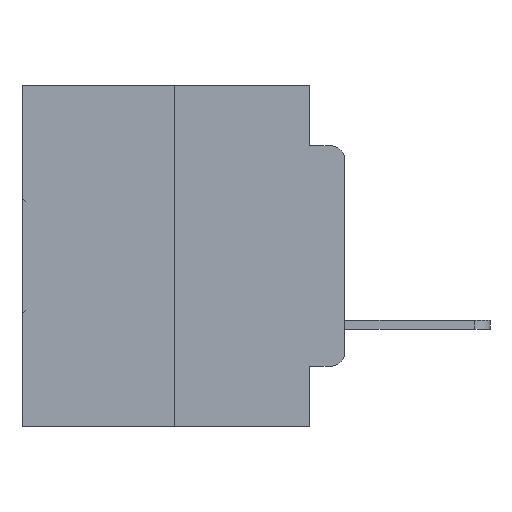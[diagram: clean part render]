
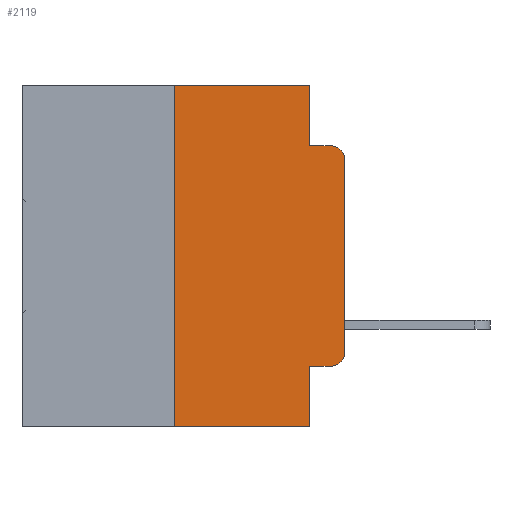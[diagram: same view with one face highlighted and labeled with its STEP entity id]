
A CAD part, left-side view. The second image highlights one B-rep face of the part: STEP entity #2119.
In plain terms, the highlighted planar face has unit normal (-1, 0, 0).
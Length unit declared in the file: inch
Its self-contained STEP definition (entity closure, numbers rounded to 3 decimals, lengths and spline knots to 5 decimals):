
#220 = EDGE_CURVE ( 'NONE', #20294, #27347, #25551, .T. ) ;
#278 = VECTOR ( 'NONE', #11086, 39.37008 ) ;
#612 = EDGE_CURVE ( 'NONE', #7777, #18776, #693, .T. ) ;
#693 = LINE ( 'NONE', #14275, #8654 ) ;
#1566 = LINE ( 'NONE', #29173, #8666 ) ;
#1867 = CARTESIAN_POINT ( 'NONE',  ( 0., 0.473, -0.5 ) ) ;
#1983 = LINE ( 'NONE', #27248, #14309 ) ;
#2119 = ADVANCED_FACE ( 'NONE', ( #10458 ), #27737, .F. ) ;
#2633 = ORIENTED_EDGE ( 'NONE', *, *, #30457, .T. ) ;
#2871 = LINE ( 'NONE', #1867, #22250 ) ;
#3010 = ORIENTED_EDGE ( 'NONE', *, *, #19916, .T. ) ;
#3434 = ORIENTED_EDGE ( 'NONE', *, *, #19320, .T. ) ;
#3666 = CIRCLE ( 'NONE', #27419, 0.02 ) ;
#3745 = CARTESIAN_POINT ( 'NONE',  ( 0., 0.25, 0. ) ) ;
#4259 = EDGE_CURVE ( 'NONE', #26759, #20294, #1566, .T. ) ;
#4433 = CARTESIAN_POINT ( 'NONE',  ( 0., 0.02, -0.1085 ) ) ;
#6158 = VERTEX_POINT ( 'NONE', #17985 ) ;
#6359 = DIRECTION ( 'NONE',  ( 0., -1., 0. ) ) ;
#6365 = ORIENTED_EDGE ( 'NONE', *, *, #220, .F. ) ;
#6709 = VERTEX_POINT ( 'NONE', #20339 ) ;
#7135 = DIRECTION ( 'NONE',  ( 0., 0., -1. ) ) ;
#7457 = CARTESIAN_POINT ( 'NONE',  ( 0., 0.051, -0.0885 ) ) ;
#7753 = DIRECTION ( 'NONE',  ( 0., 0., -1. ) ) ;
#7777 = VERTEX_POINT ( 'NONE', #27759 ) ;
#7784 = VERTEX_POINT ( 'NONE', #30035 ) ;
#8039 = ORIENTED_EDGE ( 'NONE', *, *, #15275, .T. ) ;
#8344 = DIRECTION ( 'NONE',  ( 1., 0., 0. ) ) ;
#8654 = VECTOR ( 'NONE', #7753, 39.37008 ) ;
#8666 = VECTOR ( 'NONE', #31426, 39.37008 ) ;
#10458 = FACE_OUTER_BOUND ( 'NONE', #30214, .T. ) ;
#11080 = CARTESIAN_POINT ( 'NONE',  ( 0., 0.473, 0. ) ) ;
#11086 = DIRECTION ( 'NONE',  ( 0., -1., 0. ) ) ;
#11135 = DIRECTION ( 'NONE',  ( -1., 0., 0. ) ) ;
#12658 = AXIS2_PLACEMENT_3D ( 'NONE', #23118, #8344, #25507 ) ;
#13419 = DIRECTION ( 'NONE',  ( 0., -1., 0. ) ) ;
#13485 = AXIS2_PLACEMENT_3D ( 'NONE', #4433, #22061, #7135 ) ;
#14275 = CARTESIAN_POINT ( 'NONE',  ( 0., 0.051, 0. ) ) ;
#14309 = VECTOR ( 'NONE', #29517, 39.37008 ) ;
#14893 = ORIENTED_EDGE ( 'NONE', *, *, #612, .F. ) ;
#15275 = EDGE_CURVE ( 'NONE', #26759, #18776, #2871, .T. ) ;
#15345 = VERTEX_POINT ( 'NONE', #7457 ) ;
#17192 = CARTESIAN_POINT ( 'NONE',  ( 0., 0.02, -0.4115 ) ) ;
#17556 = ORIENTED_EDGE ( 'NONE', *, *, #23241, .T. ) ;
#17985 = CARTESIAN_POINT ( 'NONE',  ( 0., 0.02, -0.0885 ) ) ;
#18318 = ORIENTED_EDGE ( 'NONE', *, *, #21848, .F. ) ;
#18385 = VECTOR ( 'NONE', #6359, 39.37008 ) ;
#18776 = VERTEX_POINT ( 'NONE', #18888 ) ;
#18888 = CARTESIAN_POINT ( 'NONE',  ( 0., 0.051, -0.5 ) ) ;
#19035 = VECTOR ( 'NONE', #25259, 39.37008 ) ;
#19320 = EDGE_CURVE ( 'NONE', #31635, #7784, #3666, .T. ) ;
#19762 = LINE ( 'NONE', #22868, #19035 ) ;
#19784 = DIRECTION ( 'NONE',  ( 0., -1., 0. ) ) ;
#19807 = ORIENTED_EDGE ( 'NONE', *, *, #4259, .F. ) ;
#19916 = EDGE_CURVE ( 'NONE', #7784, #6709, #1983, .T. ) ;
#20294 = VERTEX_POINT ( 'NONE', #3745 ) ;
#20339 = CARTESIAN_POINT ( 'NONE',  ( 0., 0., -0.1085 ) ) ;
#20689 = CARTESIAN_POINT ( 'NONE',  ( 0., 0.051, -0.4115 ) ) ;
#21848 = EDGE_CURVE ( 'NONE', #15345, #6158, #30764, .T. ) ;
#22061 = DIRECTION ( 'NONE',  ( -1., 0., 0. ) ) ;
#22250 = VECTOR ( 'NONE', #19784, 39.37008 ) ;
#22434 = CARTESIAN_POINT ( 'NONE',  ( 0., 0.051, 0. ) ) ;
#22662 = CARTESIAN_POINT ( 'NONE',  ( 0., 0.25, -0.5 ) ) ;
#22868 = CARTESIAN_POINT ( 'NONE',  ( 0., 0.051, 0. ) ) ;
#23118 = CARTESIAN_POINT ( 'NONE',  ( 0., 0.473, 0. ) ) ;
#23241 = EDGE_CURVE ( 'NONE', #6709, #6158, #29040, .T. ) ;
#23759 = CARTESIAN_POINT ( 'NONE',  ( 0., 0.051, -0.0885 ) ) ;
#25259 = DIRECTION ( 'NONE',  ( 0., 0., -1. ) ) ;
#25307 = LINE ( 'NONE', #20689, #29253 ) ;
#25507 = DIRECTION ( 'NONE',  ( 0., 0., -1. ) ) ;
#25551 = LINE ( 'NONE', #11080, #278 ) ;
#25656 = CARTESIAN_POINT ( 'NONE',  ( 0., 0.02, -0.3915 ) ) ;
#26759 = VERTEX_POINT ( 'NONE', #22662 ) ;
#27248 = CARTESIAN_POINT ( 'NONE',  ( 0., 0., 0. ) ) ;
#27347 = VERTEX_POINT ( 'NONE', #22434 ) ;
#27419 = AXIS2_PLACEMENT_3D ( 'NONE', #25656, #11135, #27979 ) ;
#27737 = PLANE ( 'NONE',  #12658 ) ;
#27759 = CARTESIAN_POINT ( 'NONE',  ( 0., 0.051, -0.4115 ) ) ;
#27979 = DIRECTION ( 'NONE',  ( 0., 0., -1. ) ) ;
#29040 = CIRCLE ( 'NONE', #13485, 0.02 ) ;
#29173 = CARTESIAN_POINT ( 'NONE',  ( 0., 0.25, 0. ) ) ;
#29253 = VECTOR ( 'NONE', #13419, 39.37008 ) ;
#29517 = DIRECTION ( 'NONE',  ( 0., 0., 1. ) ) ;
#30035 = CARTESIAN_POINT ( 'NONE',  ( 0., 0., -0.3915 ) ) ;
#30214 = EDGE_LOOP ( 'NONE', ( #3010, #17556, #18318, #30701, #6365, #19807, #8039, #14893, #2633, #3434 ) ) ;
#30387 = EDGE_CURVE ( 'NONE', #27347, #15345, #19762, .T. ) ;
#30457 = EDGE_CURVE ( 'NONE', #7777, #31635, #25307, .T. ) ;
#30701 = ORIENTED_EDGE ( 'NONE', *, *, #30387, .F. ) ;
#30764 = LINE ( 'NONE', #23759, #18385 ) ;
#31426 = DIRECTION ( 'NONE',  ( 0., 0., 1. ) ) ;
#31635 = VERTEX_POINT ( 'NONE', #17192 ) ;
